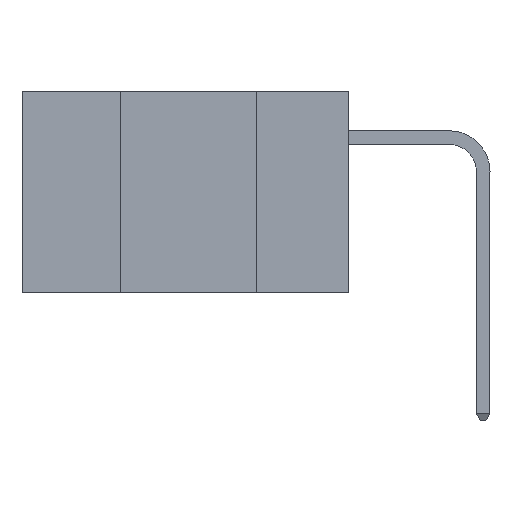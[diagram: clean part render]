
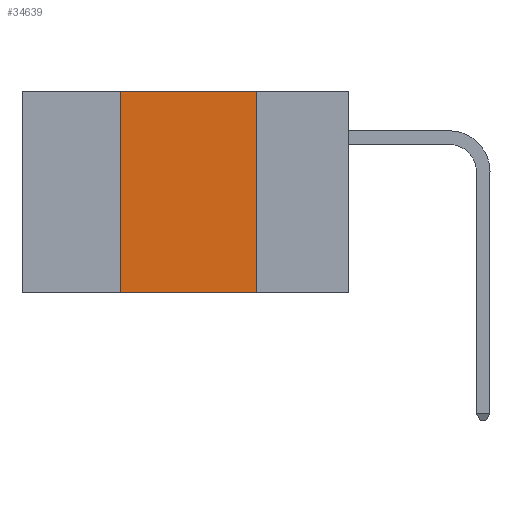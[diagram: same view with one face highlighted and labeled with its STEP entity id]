
A CAD part, left-side view. The second image highlights one B-rep face of the part: STEP entity #34639.
In plain terms, the highlighted planar face has unit normal (-1, 0, 0).
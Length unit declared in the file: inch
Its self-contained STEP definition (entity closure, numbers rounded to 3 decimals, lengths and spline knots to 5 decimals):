
#627 = DIRECTION ( 'NONE',  ( 0., -1., 0. ) ) ;
#854 = ORIENTED_EDGE ( 'NONE', *, *, #8395, .F. ) ;
#1129 = CARTESIAN_POINT ( 'NONE',  ( 0., 0.42, 0. ) ) ;
#1960 = DIRECTION ( 'NONE',  ( 0., 0., -1. ) ) ;
#2358 = VECTOR ( 'NONE', #1960, 39.37008 ) ;
#2819 = ORIENTED_EDGE ( 'NONE', *, *, #35186, .T. ) ;
#3414 = DIRECTION ( 'NONE',  ( 0., -1., 0. ) ) ;
#3697 = DIRECTION ( 'NONE',  ( 1., 0., 0. ) ) ;
#4860 = VECTOR ( 'NONE', #627, 39.37008 ) ;
#5476 = LINE ( 'NONE', #1129, #26920 ) ;
#6679 = DIRECTION ( 'NONE',  ( 0., 0., 1. ) ) ;
#7543 = VERTEX_POINT ( 'NONE', #11542 ) ;
#8395 = EDGE_CURVE ( 'NONE', #17519, #29508, #5476, .T. ) ;
#8991 = LINE ( 'NONE', #18793, #2358 ) ;
#10380 = EDGE_CURVE ( 'NONE', #29508, #7543, #10616, .T. ) ;
#10616 = LINE ( 'NONE', #17486, #4860 ) ;
#11166 = VECTOR ( 'NONE', #3414, 39.37008 ) ;
#11542 = CARTESIAN_POINT ( 'NONE',  ( 0., 0.17, 0. ) ) ;
#11757 = EDGE_LOOP ( 'NONE', ( #15624, #15042, #854, #2819 ) ) ;
#14974 = PLANE ( 'NONE',  #33155 ) ;
#15042 = ORIENTED_EDGE ( 'NONE', *, *, #10380, .F. ) ;
#15624 = ORIENTED_EDGE ( 'NONE', *, *, #16997, .F. ) ;
#16997 = EDGE_CURVE ( 'NONE', #7543, #32358, #8991, .T. ) ;
#17345 = FACE_OUTER_BOUND ( 'NONE', #11757, .T. ) ;
#17486 = CARTESIAN_POINT ( 'NONE',  ( 0., 0.6, 0. ) ) ;
#17519 = VERTEX_POINT ( 'NONE', #23782 ) ;
#18590 = LINE ( 'NONE', #28476, #11166 ) ;
#18793 = CARTESIAN_POINT ( 'NONE',  ( 0., 0.17, 0. ) ) ;
#22574 = CARTESIAN_POINT ( 'NONE',  ( 0., 0.42, 0. ) ) ;
#23375 = DIRECTION ( 'NONE',  ( 0., 0., -1. ) ) ;
#23782 = CARTESIAN_POINT ( 'NONE',  ( 0., 0.42, -0.37 ) ) ;
#26920 = VECTOR ( 'NONE', #6679, 39.37008 ) ;
#28476 = CARTESIAN_POINT ( 'NONE',  ( 0., 0.6, -0.37 ) ) ;
#28999 = CARTESIAN_POINT ( 'NONE',  ( 0., 0.17, -0.37 ) ) ;
#29508 = VERTEX_POINT ( 'NONE', #22574 ) ;
#32358 = VERTEX_POINT ( 'NONE', #28999 ) ;
#33155 = AXIS2_PLACEMENT_3D ( 'NONE', #34350, #3697, #23375 ) ;
#34350 = CARTESIAN_POINT ( 'NONE',  ( 0., 0.6, 0. ) ) ;
#34639 = ADVANCED_FACE ( 'NONE', ( #17345 ), #14974, .F. ) ;
#35186 = EDGE_CURVE ( 'NONE', #17519, #32358, #18590, .T. ) ;
